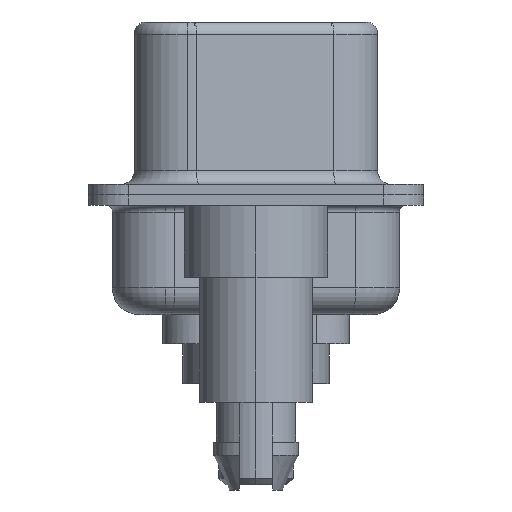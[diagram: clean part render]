
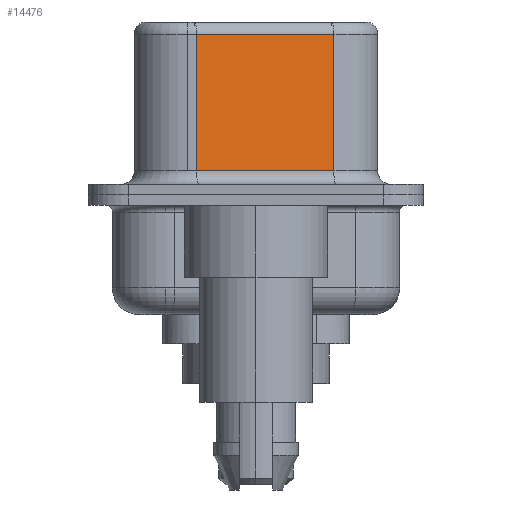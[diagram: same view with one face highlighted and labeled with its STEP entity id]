
A CAD part, left-side view. The second image highlights one B-rep face of the part: STEP entity #14476.
In plain terms, the highlighted planar face has unit normal (-0.985, -0.174, 0).
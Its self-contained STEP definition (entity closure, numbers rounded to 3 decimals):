
#344 = FACE_OUTER_BOUND ( 'NONE', #11476, .T. ) ;
#562 = ORIENTED_EDGE ( 'NONE', *, *, #16718, .T. ) ;
#1385 = LINE ( 'NONE', #4090, #7934 ) ;
#1878 = VECTOR ( 'NONE', #4743, 1000. ) ;
#2587 = CARTESIAN_POINT ( 'NONE',  ( 4.58, -2.927, 6.52 ) ) ;
#2927 = VECTOR ( 'NONE', #16771, 1000. ) ;
#3378 = EDGE_CURVE ( 'NONE', #8828, #5623, #12369, .T. ) ;
#3581 = CARTESIAN_POINT ( 'NONE',  ( 4.58, -2.927, 0.9 ) ) ;
#3738 = LINE ( 'NONE', #2587, #5586 ) ;
#3841 = DIRECTION ( 'NONE',  ( 0.985, 0.174, 0. ) ) ;
#4090 = CARTESIAN_POINT ( 'NONE',  ( 4.58, -2.927, 6.02 ) ) ;
#4295 = CARTESIAN_POINT ( 'NONE',  ( 4.58, -2.927, 6.02 ) ) ;
#4433 = EDGE_CURVE ( 'NONE', #12299, #5623, #3738, .T. ) ;
#4743 = DIRECTION ( 'NONE',  ( 0., 0., -1. ) ) ;
#5465 = CARTESIAN_POINT ( 'NONE',  ( 3.67, 2.233, 0.9 ) ) ;
#5586 = VECTOR ( 'NONE', #12952, 1000. ) ;
#5623 = VERTEX_POINT ( 'NONE', #3581 ) ;
#6080 = VERTEX_POINT ( 'NONE', #12667 ) ;
#7739 = PLANE ( 'NONE',  #13019 ) ;
#7934 = VECTOR ( 'NONE', #13213, 1000. ) ;
#8828 = VERTEX_POINT ( 'NONE', #5465 ) ;
#9061 = DIRECTION ( 'NONE',  ( -0.174, 0.985, 0. ) ) ;
#10356 = ORIENTED_EDGE ( 'NONE', *, *, #3378, .T. ) ;
#11476 = EDGE_LOOP ( 'NONE', ( #13702, #11648, #562, #10356 ) ) ;
#11648 = ORIENTED_EDGE ( 'NONE', *, *, #14437, .T. ) ;
#12299 = VERTEX_POINT ( 'NONE', #4295 ) ;
#12326 = LINE ( 'NONE', #15048, #1878 ) ;
#12369 = LINE ( 'NONE', #15372, #2927 ) ;
#12667 = CARTESIAN_POINT ( 'NONE',  ( 3.67, 2.233, 6.02 ) ) ;
#12952 = DIRECTION ( 'NONE',  ( 0., 0., -1. ) ) ;
#13019 = AXIS2_PLACEMENT_3D ( 'NONE', #15688, #3841, #9061 ) ;
#13213 = DIRECTION ( 'NONE',  ( -0.174, 0.985, 0. ) ) ;
#13702 = ORIENTED_EDGE ( 'NONE', *, *, #4433, .F. ) ;
#14437 = EDGE_CURVE ( 'NONE', #12299, #6080, #1385, .T. ) ;
#14476 = ADVANCED_FACE ( 'NONE', ( #344 ), #7739, .F. ) ;
#15048 = CARTESIAN_POINT ( 'NONE',  ( 3.67, 2.233, 6.52 ) ) ;
#15372 = CARTESIAN_POINT ( 'NONE',  ( 4.58, -2.927, 0.9 ) ) ;
#15688 = CARTESIAN_POINT ( 'NONE',  ( 4.58, -2.927, 6.52 ) ) ;
#16718 = EDGE_CURVE ( 'NONE', #6080, #8828, #12326, .T. ) ;
#16771 = DIRECTION ( 'NONE',  ( 0.174, -0.985, 0. ) ) ;
